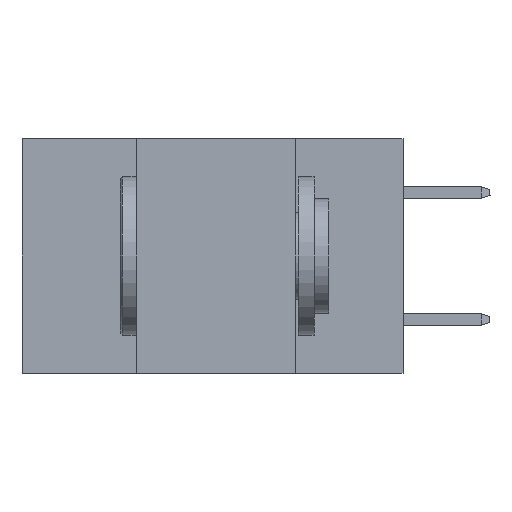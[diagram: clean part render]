
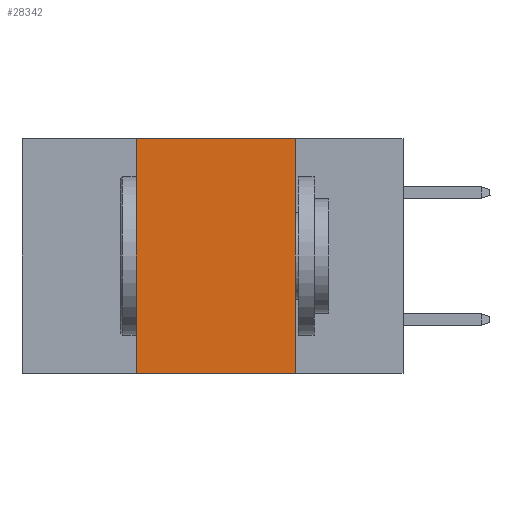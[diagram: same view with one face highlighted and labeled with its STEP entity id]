
A CAD part, left-side view. The second image highlights one B-rep face of the part: STEP entity #28342.
In plain terms, the highlighted planar face has unit normal (-1, 0, 0).
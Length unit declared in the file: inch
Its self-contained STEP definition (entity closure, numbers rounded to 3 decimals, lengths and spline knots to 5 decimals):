
#1349 = EDGE_LOOP ( 'NONE', ( #16926, #3482, #21576, #19914 ) ) ;
#1608 = VECTOR ( 'NONE', #9033, 39.37008 ) ;
#2513 = LINE ( 'NONE', #30477, #24210 ) ;
#3482 = ORIENTED_EDGE ( 'NONE', *, *, #35008, .F. ) ;
#4757 = DIRECTION ( 'NONE',  ( 1., 0., 0. ) ) ;
#4913 = EDGE_CURVE ( 'NONE', #26133, #21635, #35291, .T. ) ;
#6610 = VECTOR ( 'NONE', #26296, 39.37008 ) ;
#6990 = CARTESIAN_POINT ( 'NONE',  ( 0., 0.42, -0.37 ) ) ;
#7617 = PLANE ( 'NONE',  #20325 ) ;
#8281 = VECTOR ( 'NONE', #19235, 39.37008 ) ;
#9033 = DIRECTION ( 'NONE',  ( 0., 0., -1. ) ) ;
#16292 = VERTEX_POINT ( 'NONE', #6990 ) ;
#16561 = CARTESIAN_POINT ( 'NONE',  ( 0., 0.6, -0.37 ) ) ;
#16926 = ORIENTED_EDGE ( 'NONE', *, *, #4913, .F. ) ;
#17786 = LINE ( 'NONE', #20795, #6610 ) ;
#18475 = EDGE_CURVE ( 'NONE', #16292, #19966, #17786, .T. ) ;
#19032 = CARTESIAN_POINT ( 'NONE',  ( 0., 0.6, 0. ) ) ;
#19235 = DIRECTION ( 'NONE',  ( 0., -1., 0. ) ) ;
#19914 = ORIENTED_EDGE ( 'NONE', *, *, #26527, .T. ) ;
#19966 = VERTEX_POINT ( 'NONE', #28861 ) ;
#19971 = LINE ( 'NONE', #16561, #8281 ) ;
#20268 = CARTESIAN_POINT ( 'NONE',  ( 0., 0.17, -0.37 ) ) ;
#20325 = AXIS2_PLACEMENT_3D ( 'NONE', #19032, #4757, #27697 ) ;
#20795 = CARTESIAN_POINT ( 'NONE',  ( 0., 0.42, 0. ) ) ;
#21576 = ORIENTED_EDGE ( 'NONE', *, *, #18475, .F. ) ;
#21635 = VERTEX_POINT ( 'NONE', #20268 ) ;
#22233 = DIRECTION ( 'NONE',  ( 0., -1., 0. ) ) ;
#24210 = VECTOR ( 'NONE', #22233, 39.37008 ) ;
#26133 = VERTEX_POINT ( 'NONE', #36411 ) ;
#26296 = DIRECTION ( 'NONE',  ( 0., 0., 1. ) ) ;
#26527 = EDGE_CURVE ( 'NONE', #16292, #21635, #19971, .T. ) ;
#27697 = DIRECTION ( 'NONE',  ( 0., 0., -1. ) ) ;
#28342 = ADVANCED_FACE ( 'NONE', ( #33298 ), #7617, .F. ) ;
#28861 = CARTESIAN_POINT ( 'NONE',  ( 0., 0.42, 0. ) ) ;
#30477 = CARTESIAN_POINT ( 'NONE',  ( 0., 0.6, 0. ) ) ;
#33298 = FACE_OUTER_BOUND ( 'NONE', #1349, .T. ) ;
#34731 = CARTESIAN_POINT ( 'NONE',  ( 0., 0.17, 0. ) ) ;
#35008 = EDGE_CURVE ( 'NONE', #19966, #26133, #2513, .T. ) ;
#35291 = LINE ( 'NONE', #34731, #1608 ) ;
#36411 = CARTESIAN_POINT ( 'NONE',  ( 0., 0.17, 0. ) ) ;
